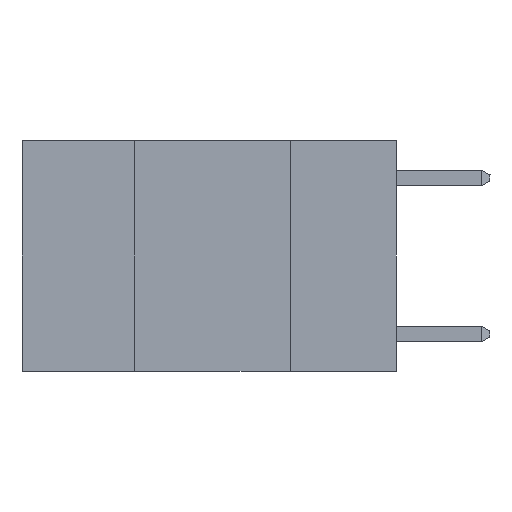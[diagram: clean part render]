
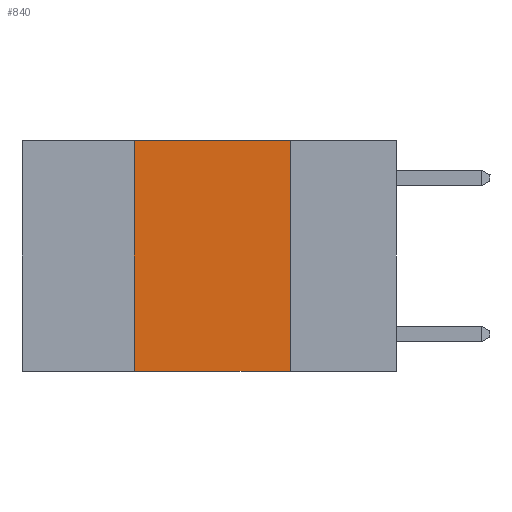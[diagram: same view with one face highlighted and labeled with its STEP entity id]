
A CAD part, left-side view. The second image highlights one B-rep face of the part: STEP entity #840.
In plain terms, the highlighted planar face has unit normal (-1, 0, 0).
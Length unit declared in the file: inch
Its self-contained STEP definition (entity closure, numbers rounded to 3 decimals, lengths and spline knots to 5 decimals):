
#198 = DIRECTION ( 'NONE',  ( 0., 0., -1. ) ) ;
#739 = VECTOR ( 'NONE', #4873, 39.37008 ) ;
#840 = ADVANCED_FACE ( 'NONE', ( #2584 ), #4262, .F. ) ;
#852 = VERTEX_POINT ( 'NONE', #5177 ) ;
#915 = DIRECTION ( 'NONE',  ( 0., 0., -1. ) ) ;
#990 = DIRECTION ( 'NONE',  ( 1., 0., 0. ) ) ;
#1178 = EDGE_CURVE ( 'NONE', #852, #6454, #1721, .T. ) ;
#1586 = ORIENTED_EDGE ( 'NONE', *, *, #1178, .F. ) ;
#1721 = LINE ( 'NONE', #8154, #5518 ) ;
#2542 = ORIENTED_EDGE ( 'NONE', *, *, #5142, .F. ) ;
#2584 = FACE_OUTER_BOUND ( 'NONE', #2819, .T. ) ;
#2685 = LINE ( 'NONE', #9169, #10250 ) ;
#2819 = EDGE_LOOP ( 'NONE', ( #1586, #2542, #8799, #8408 ) ) ;
#3174 = CARTESIAN_POINT ( 'NONE',  ( 0., 0.42, 0. ) ) ;
#4132 = CARTESIAN_POINT ( 'NONE',  ( 0., 0.17, -0.37 ) ) ;
#4262 = PLANE ( 'NONE',  #5367 ) ;
#4497 = CARTESIAN_POINT ( 'NONE',  ( 0., 0.42, 0. ) ) ;
#4506 = CARTESIAN_POINT ( 'NONE',  ( 0., 0.42, -0.37 ) ) ;
#4778 = VECTOR ( 'NONE', #5900, 39.37008 ) ;
#4873 = DIRECTION ( 'NONE',  ( 0., 0., 1. ) ) ;
#5133 = CARTESIAN_POINT ( 'NONE',  ( 0., 0.6, -0.37 ) ) ;
#5142 = EDGE_CURVE ( 'NONE', #8938, #852, #2685, .T. ) ;
#5177 = CARTESIAN_POINT ( 'NONE',  ( 0., 0.17, 0. ) ) ;
#5367 = AXIS2_PLACEMENT_3D ( 'NONE', #9869, #990, #198 ) ;
#5518 = VECTOR ( 'NONE', #915, 39.37008 ) ;
#5900 = DIRECTION ( 'NONE',  ( 0., -1., 0. ) ) ;
#5998 = LINE ( 'NONE', #5133, #4778 ) ;
#6454 = VERTEX_POINT ( 'NONE', #4132 ) ;
#6460 = LINE ( 'NONE', #3174, #739 ) ;
#7104 = EDGE_CURVE ( 'NONE', #7280, #6454, #5998, .T. ) ;
#7280 = VERTEX_POINT ( 'NONE', #4506 ) ;
#8154 = CARTESIAN_POINT ( 'NONE',  ( 0., 0.17, 0. ) ) ;
#8342 = EDGE_CURVE ( 'NONE', #7280, #8938, #6460, .T. ) ;
#8408 = ORIENTED_EDGE ( 'NONE', *, *, #7104, .T. ) ;
#8799 = ORIENTED_EDGE ( 'NONE', *, *, #8342, .F. ) ;
#8938 = VERTEX_POINT ( 'NONE', #4497 ) ;
#9007 = DIRECTION ( 'NONE',  ( 0., -1., 0. ) ) ;
#9169 = CARTESIAN_POINT ( 'NONE',  ( 0., 0.6, 0. ) ) ;
#9869 = CARTESIAN_POINT ( 'NONE',  ( 0., 0.6, 0. ) ) ;
#10250 = VECTOR ( 'NONE', #9007, 39.37008 ) ;
